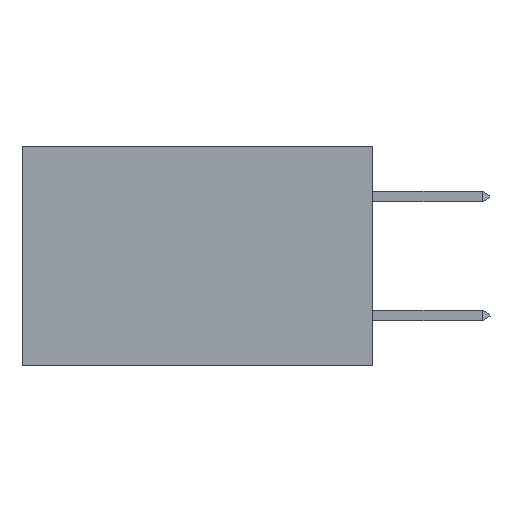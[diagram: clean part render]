
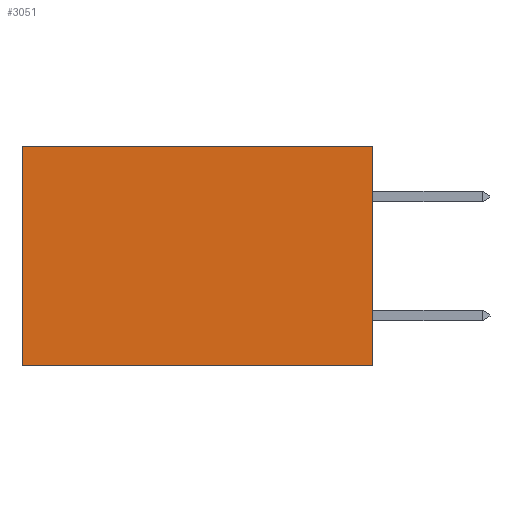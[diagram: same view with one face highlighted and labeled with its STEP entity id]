
A CAD part, left-side view. The second image highlights one B-rep face of the part: STEP entity #3051.
In plain terms, the highlighted planar face has unit normal (-1, 0, 0).
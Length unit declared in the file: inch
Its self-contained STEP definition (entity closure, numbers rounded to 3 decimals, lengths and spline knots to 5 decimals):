
#82 = ORIENTED_EDGE ( 'NONE', *, *, #8641, .F. ) ;
#1272 = DIRECTION ( 'NONE',  ( 0., 1., 0. ) ) ;
#1561 = FACE_OUTER_BOUND ( 'NONE', #7444, .T. ) ;
#1656 = LINE ( 'NONE', #5094, #5535 ) ;
#1694 = CARTESIAN_POINT ( 'NONE',  ( 0.277, 0., -0.37 ) ) ;
#2506 = VERTEX_POINT ( 'NONE', #6878 ) ;
#2741 = ORIENTED_EDGE ( 'NONE', *, *, #2836, .T. ) ;
#2836 = EDGE_CURVE ( 'NONE', #6148, #2506, #8081, .T. ) ;
#3043 = VERTEX_POINT ( 'NONE', #8664 ) ;
#3051 = ADVANCED_FACE ( 'NONE', ( #1561 ), #8674, .F. ) ;
#3959 = VECTOR ( 'NONE', #4670, 39.37008 ) ;
#4670 = DIRECTION ( 'NONE',  ( 0., 1., 0. ) ) ;
#5090 = DIRECTION ( 'NONE',  ( 0., 0., -1. ) ) ;
#5094 = CARTESIAN_POINT ( 'NONE',  ( 0.277, 0., -0.37 ) ) ;
#5306 = DIRECTION ( 'NONE',  ( 0., 0., -1. ) ) ;
#5364 = CARTESIAN_POINT ( 'NONE',  ( 0.277, 0.59, -0.37 ) ) ;
#5391 = CARTESIAN_POINT ( 'NONE',  ( 0.277, 0., 0. ) ) ;
#5535 = VECTOR ( 'NONE', #5090, 39.37008 ) ;
#5623 = VECTOR ( 'NONE', #5306, 39.37008 ) ;
#5634 = LINE ( 'NONE', #1694, #9321 ) ;
#5767 = AXIS2_PLACEMENT_3D ( 'NONE', #8019, #7937, #8059 ) ;
#6148 = VERTEX_POINT ( 'NONE', #8878 ) ;
#6464 = CARTESIAN_POINT ( 'NONE',  ( 0.277, 0.59, -0.37 ) ) ;
#6485 = ORIENTED_EDGE ( 'NONE', *, *, #9082, .T. ) ;
#6878 = CARTESIAN_POINT ( 'NONE',  ( 0.277, 0.59, 0. ) ) ;
#7107 = EDGE_CURVE ( 'NONE', #6148, #3043, #1656, .T. ) ;
#7444 = EDGE_LOOP ( 'NONE', ( #6485, #82, #8708, #2741 ) ) ;
#7937 = DIRECTION ( 'NONE',  ( 1., 0., 0. ) ) ;
#8019 = CARTESIAN_POINT ( 'NONE',  ( 0.277, 0., -0.37 ) ) ;
#8059 = DIRECTION ( 'NONE',  ( 0., 0., -1. ) ) ;
#8081 = LINE ( 'NONE', #5391, #3959 ) ;
#8501 = VERTEX_POINT ( 'NONE', #6464 ) ;
#8641 = EDGE_CURVE ( 'NONE', #3043, #8501, #5634, .T. ) ;
#8664 = CARTESIAN_POINT ( 'NONE',  ( 0.277, 0., -0.37 ) ) ;
#8674 = PLANE ( 'NONE',  #5767 ) ;
#8708 = ORIENTED_EDGE ( 'NONE', *, *, #7107, .F. ) ;
#8878 = CARTESIAN_POINT ( 'NONE',  ( 0.277, 0., 0. ) ) ;
#9082 = EDGE_CURVE ( 'NONE', #2506, #8501, #9929, .T. ) ;
#9321 = VECTOR ( 'NONE', #1272, 39.37008 ) ;
#9929 = LINE ( 'NONE', #5364, #5623 ) ;
